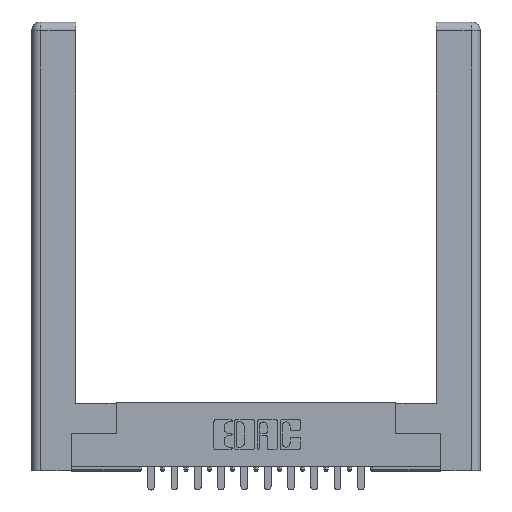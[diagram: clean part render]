
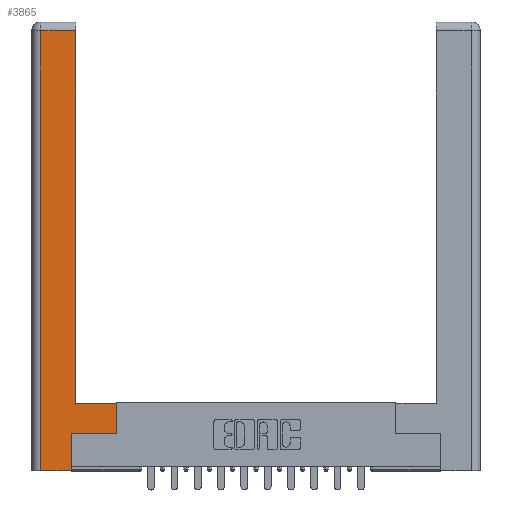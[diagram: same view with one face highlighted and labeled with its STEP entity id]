
A CAD part, top view. The second image highlights one B-rep face of the part: STEP entity #3865.
In plain terms, the highlighted planar face has unit normal (0, 0, 1).
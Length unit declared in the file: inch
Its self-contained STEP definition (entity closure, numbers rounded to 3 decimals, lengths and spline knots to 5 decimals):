
#48 = VECTOR ( 'NONE', #11961, 39.37008 ) ;
#192 = ORIENTED_EDGE ( 'NONE', *, *, #2347, .T. ) ;
#832 = EDGE_CURVE ( 'NONE', #1773, #11446, #12259, .T. ) ;
#1264 = CARTESIAN_POINT ( 'NONE',  ( 0.295, 2.94, 0. ) ) ;
#1719 = CARTESIAN_POINT ( 'NONE',  ( 0.565, 0.245, 0. ) ) ;
#1773 = VERTEX_POINT ( 'NONE', #8795 ) ;
#1955 = DIRECTION ( 'NONE',  ( 0., 0., -1. ) ) ;
#1992 = FACE_OUTER_BOUND ( 'NONE', #12142, .T. ) ;
#2347 = EDGE_CURVE ( 'NONE', #11446, #14979, #5157, .T. ) ;
#2597 = CARTESIAN_POINT ( 'NONE',  ( 0.265, 0., 0. ) ) ;
#2777 = CARTESIAN_POINT ( 'NONE',  ( 0.265, 0., 0. ) ) ;
#3243 = ORIENTED_EDGE ( 'NONE', *, *, #12568, .T. ) ;
#3800 = LINE ( 'NONE', #14654, #48 ) ;
#3865 = ADVANCED_FACE ( 'NONE', ( #1992 ), #8637, .F. ) ;
#3866 = CARTESIAN_POINT ( 'NONE',  ( 0.265, 0.245, 0. ) ) ;
#4206 = VECTOR ( 'NONE', #10682, 39.37008 ) ;
#4321 = LINE ( 'NONE', #2597, #4536 ) ;
#4536 = VECTOR ( 'NONE', #5086, 39.37008 ) ;
#4635 = ORIENTED_EDGE ( 'NONE', *, *, #832, .T. ) ;
#5038 = VECTOR ( 'NONE', #8085, 39.37008 ) ;
#5086 = DIRECTION ( 'NONE',  ( 1., 0., 0. ) ) ;
#5157 = LINE ( 'NONE', #14693, #9316 ) ;
#5602 = CARTESIAN_POINT ( 'NONE',  ( 0., 0., 0. ) ) ;
#5694 = VERTEX_POINT ( 'NONE', #13553 ) ;
#5787 = CARTESIAN_POINT ( 'NONE',  ( 0.565, 0.245, 0. ) ) ;
#6246 = EDGE_CURVE ( 'NONE', #14979, #5694, #3800, .T. ) ;
#7088 = LINE ( 'NONE', #13357, #4206 ) ;
#7108 = DIRECTION ( 'NONE',  ( 1., 0., 0. ) ) ;
#7339 = EDGE_CURVE ( 'NONE', #14153, #14590, #12177, .T. ) ;
#7509 = DIRECTION ( 'NONE',  ( -1., 0., 0. ) ) ;
#7538 = ORIENTED_EDGE ( 'NONE', *, *, #15277, .T. ) ;
#7628 = AXIS2_PLACEMENT_3D ( 'NONE', #5602, #1955, #7509 ) ;
#8085 = DIRECTION ( 'NONE',  ( 0., 1., 0. ) ) ;
#8637 = PLANE ( 'NONE',  #7628 ) ;
#8691 = DIRECTION ( 'NONE',  ( 0., -1., 0. ) ) ;
#8772 = CARTESIAN_POINT ( 'NONE',  ( 0.295, 0.45, 0. ) ) ;
#8795 = CARTESIAN_POINT ( 'NONE',  ( 0.565, 0.45, 0. ) ) ;
#9316 = VECTOR ( 'NONE', #12159, 39.37008 ) ;
#9706 = VECTOR ( 'NONE', #8691, 39.37008 ) ;
#10283 = EDGE_CURVE ( 'NONE', #14590, #1773, #12086, .T. ) ;
#10682 = DIRECTION ( 'NONE',  ( 0., 1., 0. ) ) ;
#10811 = VECTOR ( 'NONE', #12017, 39.37008 ) ;
#11446 = VERTEX_POINT ( 'NONE', #8772 ) ;
#11736 = ORIENTED_EDGE ( 'NONE', *, *, #11753, .T. ) ;
#11753 = EDGE_CURVE ( 'NONE', #14318, #14153, #7088, .T. ) ;
#11844 = CARTESIAN_POINT ( 'NONE',  ( 0.295, 0.45, 0. ) ) ;
#11961 = DIRECTION ( 'NONE',  ( -1., 0., 0. ) ) ;
#12017 = DIRECTION ( 'NONE',  ( -1., 0., 0. ) ) ;
#12086 = LINE ( 'NONE', #12119, #5038 ) ;
#12119 = CARTESIAN_POINT ( 'NONE',  ( 0.565, 0.45, 0. ) ) ;
#12142 = EDGE_LOOP ( 'NONE', ( #192, #16786, #7538, #3243, #11736, #13058, #13129, #4635 ) ) ;
#12159 = DIRECTION ( 'NONE',  ( 0., 1., 0. ) ) ;
#12177 = LINE ( 'NONE', #1719, #14712 ) ;
#12259 = LINE ( 'NONE', #11844, #10811 ) ;
#12568 = EDGE_CURVE ( 'NONE', #16935, #14318, #4321, .T. ) ;
#12595 = CARTESIAN_POINT ( 'NONE',  ( 0.0615, 0., 0. ) ) ;
#12861 = CARTESIAN_POINT ( 'NONE',  ( 0.0615, 0., 0. ) ) ;
#13058 = ORIENTED_EDGE ( 'NONE', *, *, #7339, .T. ) ;
#13129 = ORIENTED_EDGE ( 'NONE', *, *, #10283, .T. ) ;
#13357 = CARTESIAN_POINT ( 'NONE',  ( 0.265, 0.245, 0. ) ) ;
#13553 = CARTESIAN_POINT ( 'NONE',  ( 0.0615, 2.94, 0. ) ) ;
#14153 = VERTEX_POINT ( 'NONE', #3866 ) ;
#14318 = VERTEX_POINT ( 'NONE', #2777 ) ;
#14590 = VERTEX_POINT ( 'NONE', #5787 ) ;
#14654 = CARTESIAN_POINT ( 'NONE',  ( 0.0615, 2.94, 0. ) ) ;
#14693 = CARTESIAN_POINT ( 'NONE',  ( 0.295, 3., 0. ) ) ;
#14712 = VECTOR ( 'NONE', #7108, 39.37008 ) ;
#14979 = VERTEX_POINT ( 'NONE', #1264 ) ;
#15277 = EDGE_CURVE ( 'NONE', #5694, #16935, #15753, .T. ) ;
#15753 = LINE ( 'NONE', #12595, #9706 ) ;
#16786 = ORIENTED_EDGE ( 'NONE', *, *, #6246, .T. ) ;
#16935 = VERTEX_POINT ( 'NONE', #12861 ) ;
